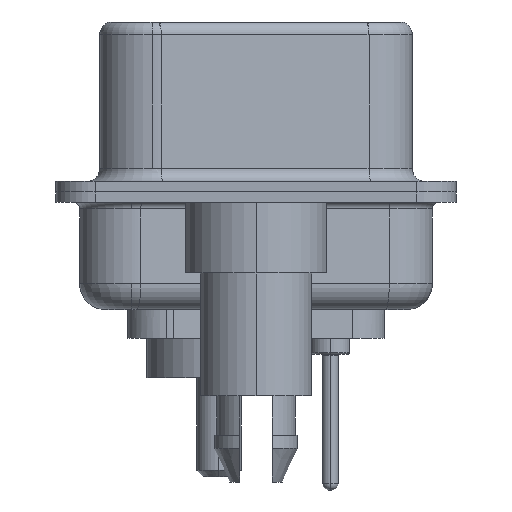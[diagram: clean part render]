
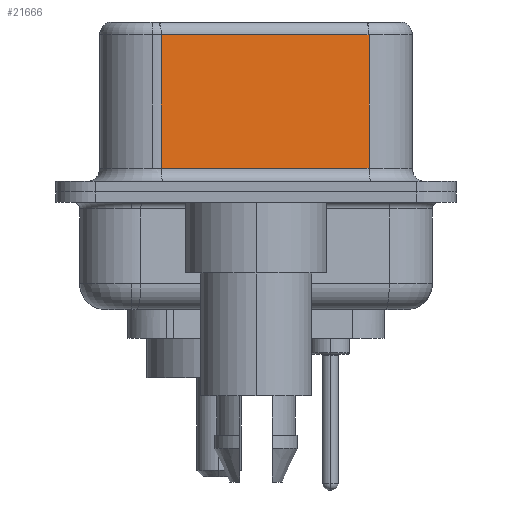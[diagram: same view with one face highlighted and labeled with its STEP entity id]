
A CAD part, left-side view. The second image highlights one B-rep face of the part: STEP entity #21666.
In plain terms, the highlighted planar face has unit normal (-0.985, -0.174, 0).
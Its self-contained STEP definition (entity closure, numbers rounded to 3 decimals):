
#231 = CARTESIAN_POINT ( 'NONE',  ( 3.73, 3.628, 6.52 ) ) ;
#326 = ORIENTED_EDGE ( 'NONE', *, *, #2861, .F. ) ;
#847 = LINE ( 'NONE', #4013, #11736 ) ;
#1609 = VERTEX_POINT ( 'NONE', #25847 ) ;
#1977 = ORIENTED_EDGE ( 'NONE', *, *, #12213, .T. ) ;
#2861 = EDGE_CURVE ( 'NONE', #24096, #18947, #21972, .T. ) ;
#3678 = VERTEX_POINT ( 'NONE', #22358 ) ;
#4013 = CARTESIAN_POINT ( 'NONE',  ( 5.132, -4.322, 0.9 ) ) ;
#4264 = CARTESIAN_POINT ( 'NONE',  ( 5.132, -4.322, 6.02 ) ) ;
#4465 = CARTESIAN_POINT ( 'NONE',  ( 5.132, -4.322, 6.02 ) ) ;
#5777 = CARTESIAN_POINT ( 'NONE',  ( 5.132, -4.322, 0.9 ) ) ;
#10257 = CARTESIAN_POINT ( 'NONE',  ( 5.132, -4.322, 6.52 ) ) ;
#10441 = DIRECTION ( 'NONE',  ( 0., 0., -1. ) ) ;
#10562 = DIRECTION ( 'NONE',  ( -0.174, 0.985, 0. ) ) ;
#11736 = VECTOR ( 'NONE', #18220, 1000. ) ;
#11829 = VECTOR ( 'NONE', #25800, 1000. ) ;
#12042 = VECTOR ( 'NONE', #10562, 1000. ) ;
#12213 = EDGE_CURVE ( 'NONE', #3678, #1609, #14253, .T. ) ;
#12252 = PLANE ( 'NONE',  #19421 ) ;
#12348 = DIRECTION ( 'NONE',  ( -0.174, 0.985, 0. ) ) ;
#13303 = LINE ( 'NONE', #4465, #12042 ) ;
#14253 = LINE ( 'NONE', #231, #23734 ) ;
#17020 = CARTESIAN_POINT ( 'NONE',  ( 5.132, -4.322, 6.52 ) ) ;
#18220 = DIRECTION ( 'NONE',  ( 0.174, -0.985, 0. ) ) ;
#18258 = EDGE_LOOP ( 'NONE', ( #326, #18858, #1977, #19954 ) ) ;
#18858 = ORIENTED_EDGE ( 'NONE', *, *, #20497, .T. ) ;
#18947 = VERTEX_POINT ( 'NONE', #5777 ) ;
#19421 = AXIS2_PLACEMENT_3D ( 'NONE', #10257, #24394, #12348 ) ;
#19954 = ORIENTED_EDGE ( 'NONE', *, *, #20305, .T. ) ;
#20305 = EDGE_CURVE ( 'NONE', #1609, #18947, #847, .T. ) ;
#20497 = EDGE_CURVE ( 'NONE', #24096, #3678, #13303, .T. ) ;
#21666 = ADVANCED_FACE ( 'NONE', ( #23976 ), #12252, .F. ) ;
#21972 = LINE ( 'NONE', #17020, #11829 ) ;
#22358 = CARTESIAN_POINT ( 'NONE',  ( 3.73, 3.628, 6.02 ) ) ;
#23734 = VECTOR ( 'NONE', #10441, 1000. ) ;
#23976 = FACE_OUTER_BOUND ( 'NONE', #18258, .T. ) ;
#24096 = VERTEX_POINT ( 'NONE', #4264 ) ;
#24394 = DIRECTION ( 'NONE',  ( 0.985, 0.174, 0. ) ) ;
#25800 = DIRECTION ( 'NONE',  ( 0., 0., -1. ) ) ;
#25847 = CARTESIAN_POINT ( 'NONE',  ( 3.73, 3.628, 0.9 ) ) ;
